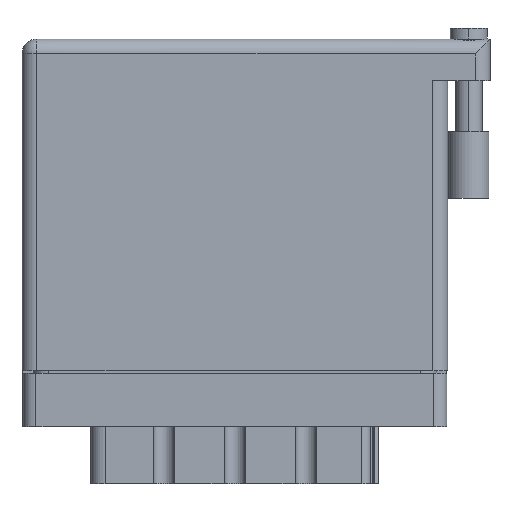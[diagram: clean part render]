
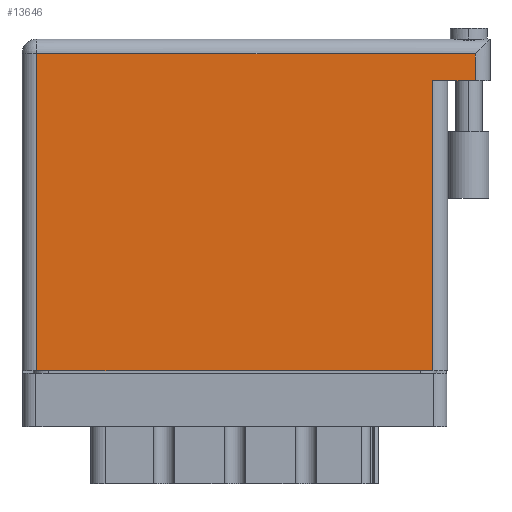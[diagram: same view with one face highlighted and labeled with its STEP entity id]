
A CAD part, front view. The second image highlights one B-rep face of the part: STEP entity #13646.
In plain terms, the highlighted face is planar.
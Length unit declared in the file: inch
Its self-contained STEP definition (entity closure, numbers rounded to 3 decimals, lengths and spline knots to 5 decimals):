
#135 = VECTOR ( 'NONE', #16147, 39.37008 ) ;
#391 = VERTEX_POINT ( 'NONE', #5017 ) ;
#3571 = CARTESIAN_POINT ( 'NONE',  ( 2.208, 1.369, 0. ) ) ;
#4590 = LINE ( 'NONE', #10213, #24797 ) ;
#5017 = CARTESIAN_POINT ( 'NONE',  ( 2.138, 1.496, 0. ) ) ;
#6637 = DIRECTION ( 'NONE',  ( -1., 0., 0. ) ) ;
#6764 = DIRECTION ( 'NONE',  ( 0., 1., 0. ) ) ;
#9301 = DIRECTION ( 'NONE',  ( -1., 0., 0. ) ) ;
#9423 = EDGE_CURVE ( 'NONE', #25338, #37712, #4590, .T. ) ;
#10039 = CARTESIAN_POINT ( 'NONE',  ( 0.07, 1.496, 0. ) ) ;
#10213 = CARTESIAN_POINT ( 'NONE',  ( 0., 0., 0. ) ) ;
#11667 = DIRECTION ( 'NONE',  ( 0., -1., 0. ) ) ;
#12998 = ORIENTED_EDGE ( 'NONE', *, *, #39440, .T. ) ;
#13534 = ORIENTED_EDGE ( 'NONE', *, *, #37731, .T. ) ;
#13646 = ADVANCED_FACE ( 'NONE', ( #39287 ), #15315, .F. ) ;
#15315 = PLANE ( 'NONE',  #19550 ) ;
#15348 = CARTESIAN_POINT ( 'NONE',  ( 2.138, 1.369, 0. ) ) ;
#16147 = DIRECTION ( 'NONE',  ( 0., 1., 0. ) ) ;
#17582 = EDGE_CURVE ( 'NONE', #391, #19915, #23108, .T. ) ;
#17659 = LINE ( 'NONE', #18079, #25097 ) ;
#18079 = CARTESIAN_POINT ( 'NONE',  ( 0.07, 0., 0. ) ) ;
#18500 = CARTESIAN_POINT ( 'NONE',  ( 0., 1.566, 0. ) ) ;
#19304 = CARTESIAN_POINT ( 'NONE',  ( 2.138, 1.566, 0. ) ) ;
#19550 = AXIS2_PLACEMENT_3D ( 'NONE', #18500, #40616, #6637 ) ;
#19915 = VERTEX_POINT ( 'NONE', #10039 ) ;
#20885 = LINE ( 'NONE', #31771, #135 ) ;
#21561 = LINE ( 'NONE', #3571, #37375 ) ;
#23108 = LINE ( 'NONE', #28262, #33001 ) ;
#24797 = VECTOR ( 'NONE', #38158, 39.37008 ) ;
#25097 = VECTOR ( 'NONE', #11667, 39.37008 ) ;
#25338 = VERTEX_POINT ( 'NONE', #28065 ) ;
#25810 = CARTESIAN_POINT ( 'NONE',  ( 1.938, 0., 0. ) ) ;
#26249 = LINE ( 'NONE', #19304, #30682 ) ;
#28065 = CARTESIAN_POINT ( 'NONE',  ( 0.07, 0., 0. ) ) ;
#28262 = CARTESIAN_POINT ( 'NONE',  ( 0., 1.496, 0. ) ) ;
#28503 = ORIENTED_EDGE ( 'NONE', *, *, #28767, .F. ) ;
#28767 = EDGE_CURVE ( 'NONE', #36933, #37042, #21561, .T. ) ;
#28936 = EDGE_LOOP ( 'NONE', ( #37396, #33593, #28503, #13534, #32620, #12998 ) ) ;
#30682 = VECTOR ( 'NONE', #6764, 39.37008 ) ;
#31254 = EDGE_CURVE ( 'NONE', #37712, #37042, #20885, .T. ) ;
#31771 = CARTESIAN_POINT ( 'NONE',  ( 1.938, 1.369, 0. ) ) ;
#32065 = CARTESIAN_POINT ( 'NONE',  ( 1.938, 1.369, 0. ) ) ;
#32620 = ORIENTED_EDGE ( 'NONE', *, *, #17582, .T. ) ;
#33001 = VECTOR ( 'NONE', #9301, 39.37008 ) ;
#33593 = ORIENTED_EDGE ( 'NONE', *, *, #31254, .T. ) ;
#36933 = VERTEX_POINT ( 'NONE', #15348 ) ;
#37042 = VERTEX_POINT ( 'NONE', #32065 ) ;
#37375 = VECTOR ( 'NONE', #38433, 39.37008 ) ;
#37396 = ORIENTED_EDGE ( 'NONE', *, *, #9423, .T. ) ;
#37712 = VERTEX_POINT ( 'NONE', #25810 ) ;
#37731 = EDGE_CURVE ( 'NONE', #36933, #391, #26249, .T. ) ;
#38158 = DIRECTION ( 'NONE',  ( 1., 0., 0. ) ) ;
#38433 = DIRECTION ( 'NONE',  ( -1., 0., 0. ) ) ;
#39287 = FACE_OUTER_BOUND ( 'NONE', #28936, .T. ) ;
#39440 = EDGE_CURVE ( 'NONE', #19915, #25338, #17659, .T. ) ;
#40616 = DIRECTION ( 'NONE',  ( 0., 0., -1. ) ) ;
